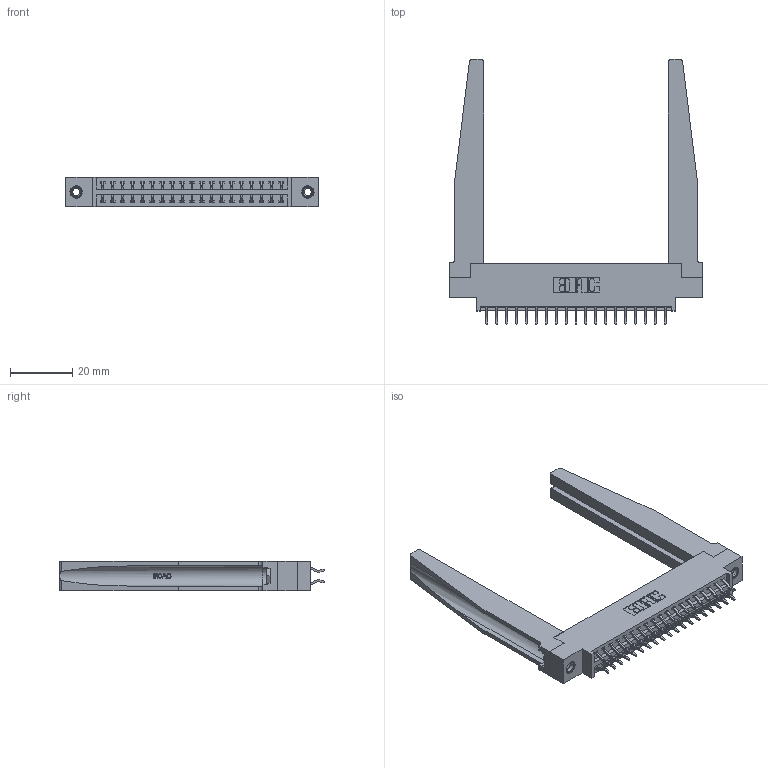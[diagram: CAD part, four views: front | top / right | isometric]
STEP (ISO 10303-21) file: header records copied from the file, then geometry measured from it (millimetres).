
FILE_DESCRIPTION (( 'STEP AP203' ), '1' );
FILE_NAME ('346-038-556-878.STEP', '2022-05-20T00:22:56', ( '' ), ( '' ), 'SwSTEP 2.0', 'SolidWorks 2020', '' );
FILE_SCHEMA (( 'CONFIG_CONTROL_DESIGN' ));
Length unit declared in the file: inch
Products named in the file (5): 345-292-001_556 Tail; 345-250-001_345-250-001-102; 346-038-556-878; 346-220-078_345-220-078; 346 Part_0.170 Offset - 0.156 Dia-TH
Assembly tree (43 placements, depth 2):
  346-038-556-878
    346 Part_0.170 Offset - 0.156 Dia-TH
    345-292-001_556 Tail  x38
    346-220-078_345-220-078  x2
    345-250-001_345-250-001-102  x2
Bounding box: 80.9 x 84.84 x 9.4 mm (x, y, z)
Volume: 14444.7 mm3; surface area: 16713.3 mm2
Topology: 43 solids, 43 shells, 2578 faces, 7559 edges, 4978 vertices
Faces by surface type: plane 1718, cylinder 808, bspline 36, cone 12, torus 4
Entity records: 21012 total; most frequent: CARTESIAN_POINT 4453, ORIENTED_EDGE 3262, DIRECTION 2949, EDGE_CURVE 1631, LINE 1321, VECTOR 1321, VERTEX_POINT 1080, AXIS2_PLACEMENT_3D 814
